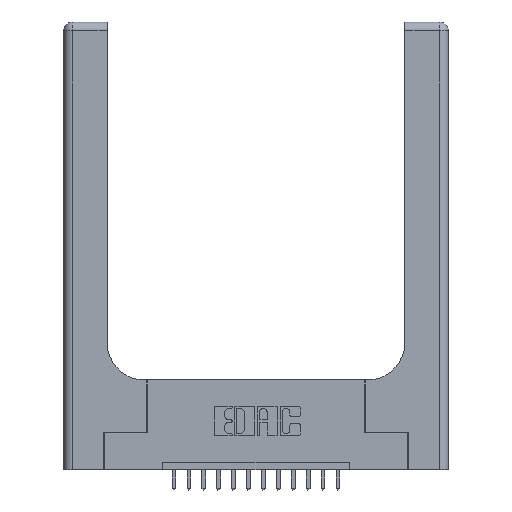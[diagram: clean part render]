
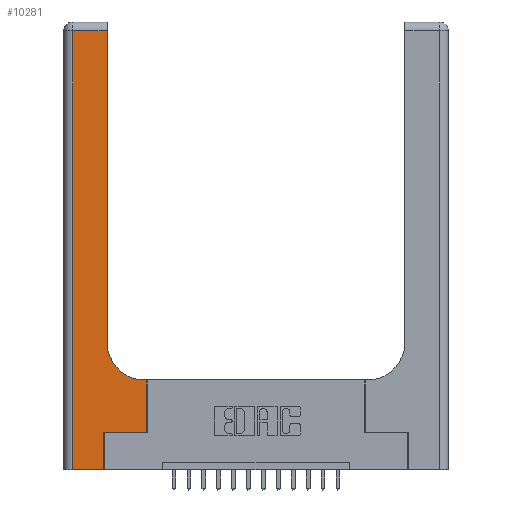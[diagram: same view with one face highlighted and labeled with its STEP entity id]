
A CAD part, top view. The second image highlights one B-rep face of the part: STEP entity #10281.
In plain terms, the highlighted planar face has unit normal (0, 0, 1).
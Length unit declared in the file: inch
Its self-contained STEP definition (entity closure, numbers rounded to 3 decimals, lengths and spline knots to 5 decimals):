
#39 = ORIENTED_EDGE ( 'NONE', *, *, #7954, .T. ) ;
#102 = EDGE_CURVE ( 'NONE', #13236, #10759, #13782, .T. ) ;
#163 = AXIS2_PLACEMENT_3D ( 'NONE', #3344, #11893, #3404 ) ;
#254 = VECTOR ( 'NONE', #15471, 39.37008 ) ;
#1132 = DIRECTION ( 'NONE',  ( -1., 0., 0. ) ) ;
#1188 = ORIENTED_EDGE ( 'NONE', *, *, #2612, .T. ) ;
#1363 = CARTESIAN_POINT ( 'NONE',  ( 0.269, 0.25, 0.37 ) ) ;
#1519 = CARTESIAN_POINT ( 'NONE',  ( 0.5585, 0.25, 0.37 ) ) ;
#1566 = LINE ( 'NONE', #13821, #10612 ) ;
#1573 = LINE ( 'NONE', #13936, #6209 ) ;
#1630 = EDGE_CURVE ( 'NONE', #14057, #11653, #17468, .T. ) ;
#1666 = VECTOR ( 'NONE', #8718, 39.37008 ) ;
#1837 = DIRECTION ( 'NONE',  ( 0., 0., -1. ) ) ;
#1883 = LINE ( 'NONE', #17967, #10260 ) ;
#2386 = EDGE_CURVE ( 'NONE', #11653, #4514, #8428, .T. ) ;
#2555 = DIRECTION ( 'NONE',  ( -1., 0., 0. ) ) ;
#2612 = EDGE_CURVE ( 'NONE', #10759, #5705, #1573, .T. ) ;
#3140 = CARTESIAN_POINT ( 'NONE',  ( 0.5415, 0.6, 0.37 ) ) ;
#3201 = DIRECTION ( 'NONE',  ( -1., 0., 0. ) ) ;
#3344 = CARTESIAN_POINT ( 'NONE',  ( 0.5415, 0.85, 0.37 ) ) ;
#3404 = DIRECTION ( 'NONE',  ( 1., 0., 0. ) ) ;
#3405 = VECTOR ( 'NONE', #15831, 39.37008 ) ;
#4034 = VECTOR ( 'NONE', #2555, 39.37008 ) ;
#4514 = VERTEX_POINT ( 'NONE', #9842 ) ;
#4748 = EDGE_CURVE ( 'NONE', #6768, #14057, #11037, .T. ) ;
#5510 = AXIS2_PLACEMENT_3D ( 'NONE', #11754, #1837, #3201 ) ;
#5539 = ORIENTED_EDGE ( 'NONE', *, *, #102, .T. ) ;
#5574 = ORIENTED_EDGE ( 'NONE', *, *, #11753, .T. ) ;
#5705 = VERTEX_POINT ( 'NONE', #14955 ) ;
#5753 = CARTESIAN_POINT ( 'NONE',  ( 0.06, 0., 0.37 ) ) ;
#5808 = VERTEX_POINT ( 'NONE', #9796 ) ;
#6209 = VECTOR ( 'NONE', #10929, 39.37008 ) ;
#6553 = EDGE_CURVE ( 'NONE', #15614, #6768, #1883, .T. ) ;
#6768 = VERTEX_POINT ( 'NONE', #7756 ) ;
#7519 = FACE_OUTER_BOUND ( 'NONE', #17022, .T. ) ;
#7591 = CARTESIAN_POINT ( 'NONE',  ( 0.269, 0.25, 0.37 ) ) ;
#7756 = CARTESIAN_POINT ( 'NONE',  ( 0.269, 0., 0.37 ) ) ;
#7954 = EDGE_CURVE ( 'NONE', #5808, #15614, #11535, .T. ) ;
#8428 = LINE ( 'NONE', #1519, #1666 ) ;
#8718 = DIRECTION ( 'NONE',  ( 0., 1., 0. ) ) ;
#8961 = DIRECTION ( 'NONE',  ( 0., 1., 0. ) ) ;
#9081 = EDGE_CURVE ( 'NONE', #5705, #5808, #15463, .T. ) ;
#9442 = ORIENTED_EDGE ( 'NONE', *, *, #2386, .T. ) ;
#9796 = CARTESIAN_POINT ( 'NONE',  ( 0.06, 2.94, 0.37 ) ) ;
#9842 = CARTESIAN_POINT ( 'NONE',  ( 0.5585, 0.6, 0.37 ) ) ;
#10006 = CARTESIAN_POINT ( 'NONE',  ( 0., 2.94, 0.37 ) ) ;
#10260 = VECTOR ( 'NONE', #13785, 39.37008 ) ;
#10281 = ADVANCED_FACE ( 'NONE', ( #7519 ), #10330, .F. ) ;
#10330 = PLANE ( 'NONE',  #5510 ) ;
#10612 = VECTOR ( 'NONE', #1132, 39.37008 ) ;
#10697 = CARTESIAN_POINT ( 'NONE',  ( 0.5585, 0.25, 0.37 ) ) ;
#10759 = VERTEX_POINT ( 'NONE', #13036 ) ;
#10929 = DIRECTION ( 'NONE',  ( 0., 1., 0. ) ) ;
#11037 = LINE ( 'NONE', #17393, #16760 ) ;
#11388 = ORIENTED_EDGE ( 'NONE', *, *, #4748, .T. ) ;
#11432 = ORIENTED_EDGE ( 'NONE', *, *, #6553, .T. ) ;
#11535 = LINE ( 'NONE', #17524, #3405 ) ;
#11653 = VERTEX_POINT ( 'NONE', #10697 ) ;
#11753 = EDGE_CURVE ( 'NONE', #4514, #13236, #1566, .T. ) ;
#11754 = CARTESIAN_POINT ( 'NONE',  ( 0., 3., 0.37 ) ) ;
#11893 = DIRECTION ( 'NONE',  ( 0., 0., -1. ) ) ;
#13036 = CARTESIAN_POINT ( 'NONE',  ( 0.2915, 0.85, 0.37 ) ) ;
#13236 = VERTEX_POINT ( 'NONE', #3140 ) ;
#13782 = CIRCLE ( 'NONE', #163, 0.25 ) ;
#13785 = DIRECTION ( 'NONE',  ( 1., 0., 0. ) ) ;
#13821 = CARTESIAN_POINT ( 'NONE',  ( 0.2915, 0.6, 0.37 ) ) ;
#13936 = CARTESIAN_POINT ( 'NONE',  ( 0.2915, 3., 0.37 ) ) ;
#14057 = VERTEX_POINT ( 'NONE', #7591 ) ;
#14955 = CARTESIAN_POINT ( 'NONE',  ( 0.2915, 2.94, 0.37 ) ) ;
#15463 = LINE ( 'NONE', #10006, #4034 ) ;
#15471 = DIRECTION ( 'NONE',  ( 1., 0., 0. ) ) ;
#15614 = VERTEX_POINT ( 'NONE', #5753 ) ;
#15831 = DIRECTION ( 'NONE',  ( 0., -1., 0. ) ) ;
#16760 = VECTOR ( 'NONE', #8961, 39.37008 ) ;
#17022 = EDGE_LOOP ( 'NONE', ( #1188, #17993, #39, #11432, #11388, #17997, #9442, #5574, #5539 ) ) ;
#17393 = CARTESIAN_POINT ( 'NONE',  ( 0.269, 0., 0.37 ) ) ;
#17468 = LINE ( 'NONE', #1363, #254 ) ;
#17524 = CARTESIAN_POINT ( 'NONE',  ( 0.06, 3., 0.37 ) ) ;
#17967 = CARTESIAN_POINT ( 'NONE',  ( 0., 0., 0.37 ) ) ;
#17993 = ORIENTED_EDGE ( 'NONE', *, *, #9081, .T. ) ;
#17997 = ORIENTED_EDGE ( 'NONE', *, *, #1630, .T. ) ;
